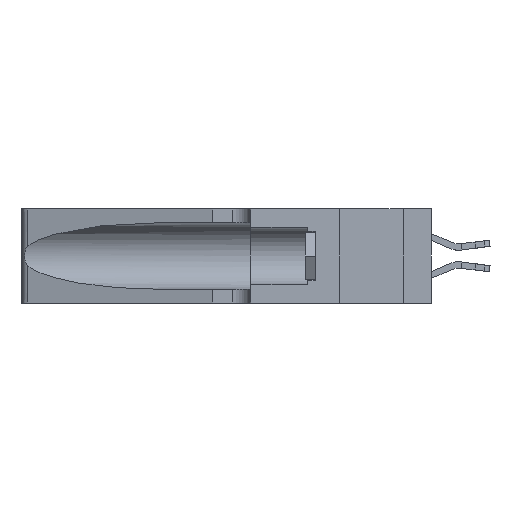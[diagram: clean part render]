
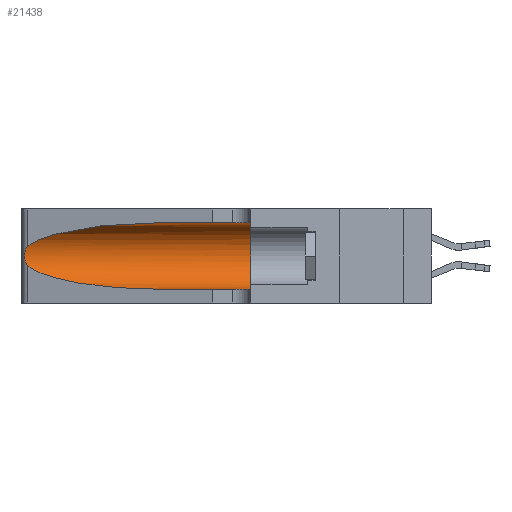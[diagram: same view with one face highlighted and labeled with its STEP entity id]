
A CAD part, left-side view. The second image highlights one B-rep face of the part: STEP entity #21438.
In plain terms, the highlighted cylindrical face has radius 3.308 mm (diameter 6.617 mm), a partial arc.
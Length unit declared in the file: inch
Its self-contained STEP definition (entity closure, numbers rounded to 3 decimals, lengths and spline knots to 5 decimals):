
#394 = EDGE_CURVE ( 'NONE', #3717, #24894, #16537, .T. ) ;
#2037 = CARTESIAN_POINT ( 'NONE',  ( 0.26075, 1.23896, 0.178 ) ) ;
#2641 = DIRECTION ( 'NONE',  ( 0., -1., 0. ) ) ;
#3175 = AXIS2_PLACEMENT_3D ( 'NONE', #19490, #27269, #22255 ) ;
#3493 = LINE ( 'NONE', #35449, #33174 ) ;
#3717 = VERTEX_POINT ( 'NONE', #21544 ) ;
#3749 = VERTEX_POINT ( 'NONE', #24290 ) ;
#4292 = EDGE_CURVE ( 'NONE', #3717, #26915, #23947, .T. ) ;
#4422 = CARTESIAN_POINT ( 'NONE',  ( 0.25487, 1.22718, 0.22369 ) ) ;
#4891 = CARTESIAN_POINT ( 'NONE',  ( 0.1305, 0.72297, 0.31525 ) ) ;
#6830 = CARTESIAN_POINT ( 'NONE',  ( 0.1305, 0.35, 0.31525 ) ) ;
#7191 = CARTESIAN_POINT ( 'NONE',  ( 0.25555, 1.22994, 0.2215 ) ) ;
#7436 = CARTESIAN_POINT ( 'NONE',  ( 0.25854, 1.2359, 0.20912 ) ) ;
#7624 = CARTESIAN_POINT ( 'NONE',  ( 0.1305, 1.61858, 0.31525 ) ) ;
#8623 = CARTESIAN_POINT ( 'NONE',  ( 0.2373, 1.15595, 0.08982 ) ) ;
#8687 = ORIENTED_EDGE ( 'NONE', *, *, #12748, .T. ) ;
#10384 = EDGE_CURVE ( 'NONE', #26915, #12920, #26022, .T. ) ;
#12748 = EDGE_CURVE ( 'NONE', #3749, #28894, #17613, .T. ) ;
#12820 = CARTESIAN_POINT ( 'NONE',  ( 0.1305, 0.72297, 0.05475 ) ) ;
#12920 = VERTEX_POINT ( 'NONE', #22414 ) ;
#12993 = CARTESIAN_POINT ( 'NONE',  ( 0.26017, 1.23833, 0.17102 ) ) ;
#13042 = ORIENTED_EDGE ( 'NONE', *, *, #10384, .F. ) ;
#13136 = ORIENTED_EDGE ( 'NONE', *, *, #27653, .T. ) ;
#13184 = DIRECTION ( 'NONE',  ( 0., -1., 0. ) ) ;
#13634 = EDGE_LOOP ( 'NONE', ( #26552, #29794, #8687, #13136, #13042, #16388 ) ) ;
#13862 = DIRECTION ( 'NONE',  ( 0., -1., 0. ) ) ;
#14169 = CARTESIAN_POINT ( 'NONE',  ( 0.18966, 0.96281, 0.05475 ) ) ;
#16388 = ORIENTED_EDGE ( 'NONE', *, *, #4292, .F. ) ;
#16537 =( BOUNDED_CURVE ( )  B_SPLINE_CURVE ( 3, ( #4891, #34917, #18332, #32019 ),
 .UNSPECIFIED., .F., .T. ) 
 B_SPLINE_CURVE_WITH_KNOTS ( ( 4, 4 ),
 ( 1.5708, 2.84003 ),
 .UNSPECIFIED. ) 
 CURVE ( )  GEOMETRIC_REPRESENTATION_ITEM ( )  RATIONAL_B_SPLINE_CURVE ( ( 1., 0.87, 0.87, 1. ) ) 
 REPRESENTATION_ITEM ( '' )  );
#16598 = VECTOR ( 'NONE', #13862, 39.37008 ) ;
#17613 =( BOUNDED_CURVE ( )  B_SPLINE_CURVE ( 3, ( #27499, #8623, #14169, #33031 ),
 .UNSPECIFIED., .F., .F. ) 
 B_SPLINE_CURVE_WITH_KNOTS ( ( 4, 4 ),
 ( 3.44316, 4.71239 ),
 .UNSPECIFIED. ) 
 CURVE ( )  GEOMETRIC_REPRESENTATION_ITEM ( )  RATIONAL_B_SPLINE_CURVE ( ( 1., 0.87, 0.87, 1. ) ) 
 REPRESENTATION_ITEM ( '' )  );
#18332 = CARTESIAN_POINT ( 'NONE',  ( 0.2373, 1.15595, 0.28018 ) ) ;
#18760 = B_SPLINE_CURVE_WITH_KNOTS ( 'NONE', 3,
 ( #4422, #7191, #35333, #35214, #7436, #32055, #29523, #2037, #12993, #26891, #34832, #32424, #32177, #21673 ),
 .UNSPECIFIED., .F., .F.,
 ( 4, 2, 2, 2, 2, 2, 4 ),
 ( 0., 0.00027, 0.00053, 0.00107, 0.0016, 0.00187, 0.00214 ),
 .UNSPECIFIED. ) ;
#19490 = CARTESIAN_POINT ( 'NONE',  ( 0.1305, 0.35, 0.185 ) ) ;
#20997 = CARTESIAN_POINT ( 'NONE',  ( 0.1305, 1.61858, 0.185 ) ) ;
#21438 = ADVANCED_FACE ( 'NONE', ( #27079 ), #28770, .F. ) ;
#21544 = CARTESIAN_POINT ( 'NONE',  ( 0.1305, 0.72297, 0.31525 ) ) ;
#21673 = CARTESIAN_POINT ( 'NONE',  ( 0.25487, 1.22718, 0.14631 ) ) ;
#22255 = DIRECTION ( 'NONE',  ( 0., 0., 1. ) ) ;
#22414 = CARTESIAN_POINT ( 'NONE',  ( 0.1305, 0.35, 0.05475 ) ) ;
#23947 = LINE ( 'NONE', #7624, #16598 ) ;
#24290 = CARTESIAN_POINT ( 'NONE',  ( 0.25487, 1.22718, 0.14631 ) ) ;
#24894 = VERTEX_POINT ( 'NONE', #30060 ) ;
#25034 = AXIS2_PLACEMENT_3D ( 'NONE', #20997, #13184, #29352 ) ;
#25263 = EDGE_CURVE ( 'NONE', #24894, #3749, #18760, .T. ) ;
#26022 = CIRCLE ( 'NONE', #3175, 0.13025 ) ;
#26552 = ORIENTED_EDGE ( 'NONE', *, *, #394, .T. ) ;
#26891 = CARTESIAN_POINT ( 'NONE',  ( 0.25856, 1.23593, 0.16098 ) ) ;
#26915 = VERTEX_POINT ( 'NONE', #6830 ) ;
#27079 = FACE_OUTER_BOUND ( 'NONE', #13634, .T. ) ;
#27269 = DIRECTION ( 'NONE',  ( 0., 1., 0. ) ) ;
#27499 = CARTESIAN_POINT ( 'NONE',  ( 0.25487, 1.22718, 0.14631 ) ) ;
#27653 = EDGE_CURVE ( 'NONE', #28894, #12920, #3493, .T. ) ;
#28770 = CYLINDRICAL_SURFACE ( 'NONE', #25034, 0.13025 ) ;
#28894 = VERTEX_POINT ( 'NONE', #12820 ) ;
#29352 = DIRECTION ( 'NONE',  ( 0., 0., -1. ) ) ;
#29523 = CARTESIAN_POINT ( 'NONE',  ( 0.26075, 1.23896, 0.19203 ) ) ;
#29794 = ORIENTED_EDGE ( 'NONE', *, *, #25263, .T. ) ;
#30060 = CARTESIAN_POINT ( 'NONE',  ( 0.25487, 1.22718, 0.22369 ) ) ;
#32019 = CARTESIAN_POINT ( 'NONE',  ( 0.25487, 1.22718, 0.22369 ) ) ;
#32055 = CARTESIAN_POINT ( 'NONE',  ( 0.26018, 1.23835, 0.19895 ) ) ;
#32177 = CARTESIAN_POINT ( 'NONE',  ( 0.25555, 1.22993, 0.14849 ) ) ;
#32424 = CARTESIAN_POINT ( 'NONE',  ( 0.25639, 1.23186, 0.15144 ) ) ;
#33031 = CARTESIAN_POINT ( 'NONE',  ( 0.1305, 0.72297, 0.05475 ) ) ;
#33174 = VECTOR ( 'NONE', #2641, 39.37008 ) ;
#34832 = CARTESIAN_POINT ( 'NONE',  ( 0.25789, 1.23486, 0.15765 ) ) ;
#34917 = CARTESIAN_POINT ( 'NONE',  ( 0.18966, 0.96281, 0.31525 ) ) ;
#35214 = CARTESIAN_POINT ( 'NONE',  ( 0.25787, 1.23484, 0.2124 ) ) ;
#35333 = CARTESIAN_POINT ( 'NONE',  ( 0.25639, 1.23184, 0.21858 ) ) ;
#35449 = CARTESIAN_POINT ( 'NONE',  ( 0.1305, 1.61858, 0.05475 ) ) ;
